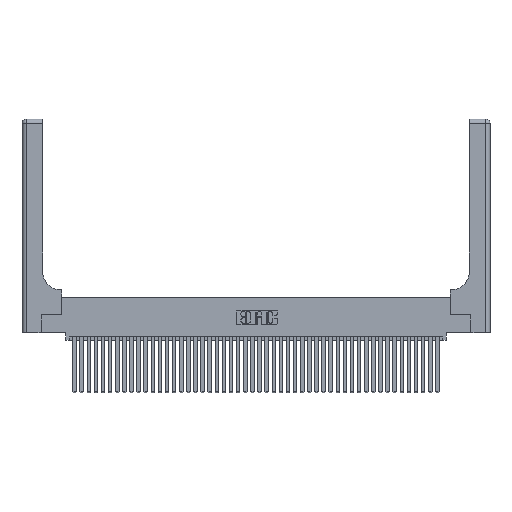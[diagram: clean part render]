
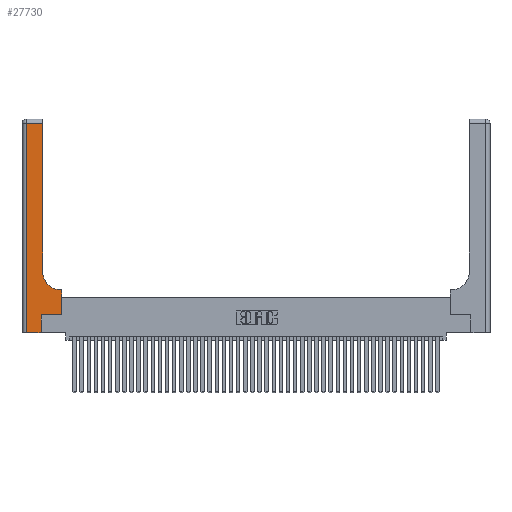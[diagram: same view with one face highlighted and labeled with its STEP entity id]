
A CAD part, top view. The second image highlights one B-rep face of the part: STEP entity #27730.
In plain terms, the highlighted planar face has unit normal (0, 0, 1).
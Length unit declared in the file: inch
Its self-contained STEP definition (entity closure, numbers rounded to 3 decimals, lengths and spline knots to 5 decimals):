
#260 = DIRECTION ( 'NONE',  ( -1., 0., 0. ) ) ;
#454 = EDGE_CURVE ( 'NONE', #23850, #40889, #32598, .T. ) ;
#1158 = VERTEX_POINT ( 'NONE', #36978 ) ;
#1177 = CARTESIAN_POINT ( 'NONE',  ( 0.2915, 0.85, 0.37 ) ) ;
#2516 = DIRECTION ( 'NONE',  ( -1., 0., 0. ) ) ;
#3668 = EDGE_CURVE ( 'NONE', #19686, #29484, #34496, .T. ) ;
#4452 = ORIENTED_EDGE ( 'NONE', *, *, #20434, .T. ) ;
#5770 = DIRECTION ( 'NONE',  ( 0., 1., 0. ) ) ;
#5979 = CARTESIAN_POINT ( 'NONE',  ( 0., 0., 0.37 ) ) ;
#6449 = VERTEX_POINT ( 'NONE', #6708 ) ;
#6683 = ORIENTED_EDGE ( 'NONE', *, *, #3668, .T. ) ;
#6708 = CARTESIAN_POINT ( 'NONE',  ( 0.269, 0., 0.37 ) ) ;
#6952 = VECTOR ( 'NONE', #260, 39.37008 ) ;
#7680 = VERTEX_POINT ( 'NONE', #12461 ) ;
#9225 = DIRECTION ( 'NONE',  ( 1., 0., 0. ) ) ;
#10183 = VECTOR ( 'NONE', #38551, 39.37008 ) ;
#10393 = ORIENTED_EDGE ( 'NONE', *, *, #10880, .T. ) ;
#10880 = EDGE_CURVE ( 'NONE', #7680, #6449, #16640, .T. ) ;
#11154 = CARTESIAN_POINT ( 'NONE',  ( 0.269, 0., 0.37 ) ) ;
#12461 = CARTESIAN_POINT ( 'NONE',  ( 0.06, 0., 0.37 ) ) ;
#13887 = VERTEX_POINT ( 'NONE', #17882 ) ;
#14121 = CARTESIAN_POINT ( 'NONE',  ( 0.06, 2.94, 0.37 ) ) ;
#14438 = CARTESIAN_POINT ( 'NONE',  ( 0.5585, 0.25, 0.37 ) ) ;
#14593 = DIRECTION ( 'NONE',  ( 0., 1., 0. ) ) ;
#15128 = DIRECTION ( 'NONE',  ( 0., -1., 0. ) ) ;
#15920 = DIRECTION ( 'NONE',  ( 0., 0., -1. ) ) ;
#16281 = AXIS2_PLACEMENT_3D ( 'NONE', #36593, #15920, #40027 ) ;
#16404 = ORIENTED_EDGE ( 'NONE', *, *, #33566, .T. ) ;
#16580 = ORIENTED_EDGE ( 'NONE', *, *, #31158, .T. ) ;
#16640 = LINE ( 'NONE', #5979, #33929 ) ;
#17882 = CARTESIAN_POINT ( 'NONE',  ( 0.5585, 0.25, 0.37 ) ) ;
#18229 = LINE ( 'NONE', #14438, #10183 ) ;
#18610 = EDGE_CURVE ( 'NONE', #6449, #19034, #41395, .T. ) ;
#19034 = VERTEX_POINT ( 'NONE', #37366 ) ;
#19686 = VERTEX_POINT ( 'NONE', #35550 ) ;
#19690 = PLANE ( 'NONE',  #21544 ) ;
#20434 = EDGE_CURVE ( 'NONE', #29484, #7680, #40763, .T. ) ;
#20798 = LINE ( 'NONE', #22956, #36977 ) ;
#21544 = AXIS2_PLACEMENT_3D ( 'NONE', #43780, #23183, #2516 ) ;
#21705 = ORIENTED_EDGE ( 'NONE', *, *, #18610, .T. ) ;
#22245 = CARTESIAN_POINT ( 'NONE',  ( 0.5415, 0.6, 0.37 ) ) ;
#22535 = FACE_OUTER_BOUND ( 'NONE', #27231, .T. ) ;
#22803 = CARTESIAN_POINT ( 'NONE',  ( 0.269, 0.25, 0.37 ) ) ;
#22956 = CARTESIAN_POINT ( 'NONE',  ( 0.2915, 3., 0.37 ) ) ;
#23183 = DIRECTION ( 'NONE',  ( 0., 0., -1. ) ) ;
#23749 = LINE ( 'NONE', #31060, #40997 ) ;
#23850 = VERTEX_POINT ( 'NONE', #22245 ) ;
#24403 = CARTESIAN_POINT ( 'NONE',  ( 0., 2.94, 0.37 ) ) ;
#27231 = EDGE_LOOP ( 'NONE', ( #16404, #6683, #4452, #10393, #21705, #33860, #39201, #16580, #43876 ) ) ;
#27361 = EDGE_CURVE ( 'NONE', #13887, #1158, #18229, .T. ) ;
#27730 = ADVANCED_FACE ( 'NONE', ( #22535 ), #19690, .F. ) ;
#28895 = VECTOR ( 'NONE', #9225, 39.37008 ) ;
#29484 = VERTEX_POINT ( 'NONE', #14121 ) ;
#30123 = DIRECTION ( 'NONE',  ( 1., 0., 0. ) ) ;
#31060 = CARTESIAN_POINT ( 'NONE',  ( 0.2915, 0.6, 0.37 ) ) ;
#31158 = EDGE_CURVE ( 'NONE', #1158, #23850, #23749, .T. ) ;
#31600 = VECTOR ( 'NONE', #15128, 39.37008 ) ;
#32242 = VECTOR ( 'NONE', #14593, 39.37008 ) ;
#32598 = CIRCLE ( 'NONE', #16281, 0.25 ) ;
#33558 = EDGE_CURVE ( 'NONE', #19034, #13887, #38054, .T. ) ;
#33566 = EDGE_CURVE ( 'NONE', #40889, #19686, #20798, .T. ) ;
#33860 = ORIENTED_EDGE ( 'NONE', *, *, #33558, .T. ) ;
#33929 = VECTOR ( 'NONE', #30123, 39.37008 ) ;
#34496 = LINE ( 'NONE', #24403, #6952 ) ;
#35550 = CARTESIAN_POINT ( 'NONE',  ( 0.2915, 2.94, 0.37 ) ) ;
#35798 = CARTESIAN_POINT ( 'NONE',  ( 0.06, 3., 0.37 ) ) ;
#36593 = CARTESIAN_POINT ( 'NONE',  ( 0.5415, 0.85, 0.37 ) ) ;
#36977 = VECTOR ( 'NONE', #5770, 39.37008 ) ;
#36978 = CARTESIAN_POINT ( 'NONE',  ( 0.5585, 0.6, 0.37 ) ) ;
#37366 = CARTESIAN_POINT ( 'NONE',  ( 0.269, 0.25, 0.37 ) ) ;
#37967 = DIRECTION ( 'NONE',  ( -1., 0., 0. ) ) ;
#38054 = LINE ( 'NONE', #22803, #28895 ) ;
#38551 = DIRECTION ( 'NONE',  ( 0., 1., 0. ) ) ;
#39201 = ORIENTED_EDGE ( 'NONE', *, *, #27361, .T. ) ;
#40027 = DIRECTION ( 'NONE',  ( 1., 0., 0. ) ) ;
#40763 = LINE ( 'NONE', #35798, #31600 ) ;
#40889 = VERTEX_POINT ( 'NONE', #1177 ) ;
#40997 = VECTOR ( 'NONE', #37967, 39.37008 ) ;
#41395 = LINE ( 'NONE', #11154, #32242 ) ;
#43780 = CARTESIAN_POINT ( 'NONE',  ( 0., 3., 0.37 ) ) ;
#43876 = ORIENTED_EDGE ( 'NONE', *, *, #454, .T. ) ;
